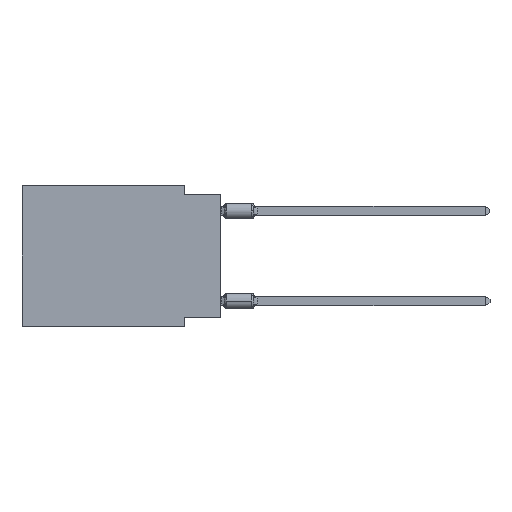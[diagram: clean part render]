
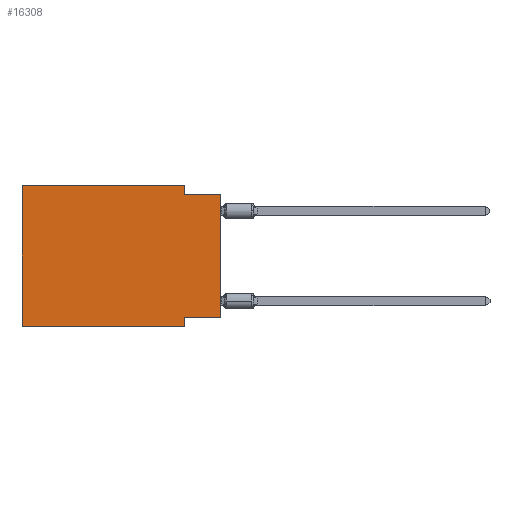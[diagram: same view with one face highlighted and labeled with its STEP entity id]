
A CAD part, left-side view. The second image highlights one B-rep face of the part: STEP entity #16308.
In plain terms, the highlighted planar face has unit normal (-1, 0, 0).
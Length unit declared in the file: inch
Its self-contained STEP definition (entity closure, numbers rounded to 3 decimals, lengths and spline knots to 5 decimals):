
#1182 = VERTEX_POINT ( 'NONE', #14767 ) ;
#1268 = AXIS2_PLACEMENT_3D ( 'NONE', #7050, #26869, #10856 ) ;
#2631 = DIRECTION ( 'NONE',  ( 0., 0., -1. ) ) ;
#3006 = EDGE_CURVE ( 'NONE', #36230, #23345, #48469, .T. ) ;
#3013 = LINE ( 'NONE', #48326, #14189 ) ;
#3287 = CARTESIAN_POINT ( 'NONE',  ( 0., 0.1, -0.39 ) ) ;
#4410 = CARTESIAN_POINT ( 'NONE',  ( 0., 0.1, -0.025 ) ) ;
#4413 = ORIENTED_EDGE ( 'NONE', *, *, #25421, .F. ) ;
#4939 = DIRECTION ( 'NONE',  ( 0., -1., 0. ) ) ;
#4994 = VERTEX_POINT ( 'NONE', #48086 ) ;
#7050 = CARTESIAN_POINT ( 'NONE',  ( 0., 0.55, 0. ) ) ;
#7879 = ORIENTED_EDGE ( 'NONE', *, *, #24245, .F. ) ;
#8689 = CARTESIAN_POINT ( 'NONE',  ( 0., 0.55, -0.39 ) ) ;
#9275 = CARTESIAN_POINT ( 'NONE',  ( 0., 0., -0.365 ) ) ;
#10856 = DIRECTION ( 'NONE',  ( 0., 0., -1. ) ) ;
#10916 = VECTOR ( 'NONE', #2631, 39.37008 ) ;
#11179 = CARTESIAN_POINT ( 'NONE',  ( 0., 0.1, -0.39 ) ) ;
#14189 = VECTOR ( 'NONE', #52661, 39.37008 ) ;
#14614 = VERTEX_POINT ( 'NONE', #11179 ) ;
#14627 = EDGE_LOOP ( 'NONE', ( #42340, #7879, #46774, #4413, #25783, #42795, #32193, #40456 ) ) ;
#14767 = CARTESIAN_POINT ( 'NONE',  ( 0., 0., -0.365 ) ) ;
#16308 = ADVANCED_FACE ( 'NONE', ( #47497 ), #23058, .F. ) ;
#16855 = DIRECTION ( 'NONE',  ( 0., 1., 0. ) ) ;
#17126 = LINE ( 'NONE', #9275, #35030 ) ;
#19796 = EDGE_CURVE ( 'NONE', #1182, #48829, #17126, .T. ) ;
#21618 = LINE ( 'NONE', #33315, #40426 ) ;
#23058 = PLANE ( 'NONE',  #1268 ) ;
#23190 = DIRECTION ( 'NONE',  ( 0., 0., 1. ) ) ;
#23345 = VERTEX_POINT ( 'NONE', #4410 ) ;
#24245 = EDGE_CURVE ( 'NONE', #23345, #4994, #21618, .T. ) ;
#24472 = VECTOR ( 'NONE', #49923, 39.37008 ) ;
#24552 = VERTEX_POINT ( 'NONE', #31359 ) ;
#25267 = LINE ( 'NONE', #42107, #45704 ) ;
#25421 = EDGE_CURVE ( 'NONE', #49332, #36230, #25267, .T. ) ;
#25695 = DIRECTION ( 'NONE',  ( 0., -1., 0. ) ) ;
#25783 = ORIENTED_EDGE ( 'NONE', *, *, #34058, .F. ) ;
#26869 = DIRECTION ( 'NONE',  ( 1., 0., 0. ) ) ;
#27045 = CARTESIAN_POINT ( 'NONE',  ( 0., 0.1, 0. ) ) ;
#28345 = LINE ( 'NONE', #44614, #34108 ) ;
#28780 = DIRECTION ( 'NONE',  ( 0., 0., -1. ) ) ;
#29845 = LINE ( 'NONE', #8689, #24472 ) ;
#31359 = CARTESIAN_POINT ( 'NONE',  ( 0., 0.55, -0.39 ) ) ;
#32193 = ORIENTED_EDGE ( 'NONE', *, *, #51694, .F. ) ;
#33315 = CARTESIAN_POINT ( 'NONE',  ( 0., 0., -0.025 ) ) ;
#34058 = EDGE_CURVE ( 'NONE', #24552, #49332, #28345, .T. ) ;
#34108 = VECTOR ( 'NONE', #23190, 39.37008 ) ;
#35030 = VECTOR ( 'NONE', #16855, 39.37008 ) ;
#36230 = VERTEX_POINT ( 'NONE', #52368 ) ;
#36698 = CARTESIAN_POINT ( 'NONE',  ( 0., 0.1, -0.365 ) ) ;
#40426 = VECTOR ( 'NONE', #25695, 39.37008 ) ;
#40453 = LINE ( 'NONE', #3287, #51501 ) ;
#40456 = ORIENTED_EDGE ( 'NONE', *, *, #19796, .F. ) ;
#42107 = CARTESIAN_POINT ( 'NONE',  ( 0., 0.55, 0. ) ) ;
#42340 = ORIENTED_EDGE ( 'NONE', *, *, #51646, .T. ) ;
#42795 = ORIENTED_EDGE ( 'NONE', *, *, #50523, .T. ) ;
#44614 = CARTESIAN_POINT ( 'NONE',  ( 0., 0.55, 0. ) ) ;
#45704 = VECTOR ( 'NONE', #4939, 39.37008 ) ;
#46774 = ORIENTED_EDGE ( 'NONE', *, *, #3006, .F. ) ;
#47497 = FACE_OUTER_BOUND ( 'NONE', #14627, .T. ) ;
#48086 = CARTESIAN_POINT ( 'NONE',  ( 0., 0., -0.025 ) ) ;
#48326 = CARTESIAN_POINT ( 'NONE',  ( 0., 0., 0. ) ) ;
#48469 = LINE ( 'NONE', #27045, #10916 ) ;
#48829 = VERTEX_POINT ( 'NONE', #36698 ) ;
#49332 = VERTEX_POINT ( 'NONE', #53438 ) ;
#49923 = DIRECTION ( 'NONE',  ( 0., -1., 0. ) ) ;
#50523 = EDGE_CURVE ( 'NONE', #24552, #14614, #29845, .T. ) ;
#51501 = VECTOR ( 'NONE', #28780, 39.37008 ) ;
#51646 = EDGE_CURVE ( 'NONE', #1182, #4994, #3013, .T. ) ;
#51694 = EDGE_CURVE ( 'NONE', #48829, #14614, #40453, .T. ) ;
#52368 = CARTESIAN_POINT ( 'NONE',  ( 0., 0.1, 0. ) ) ;
#52661 = DIRECTION ( 'NONE',  ( 0., 0., 1. ) ) ;
#53438 = CARTESIAN_POINT ( 'NONE',  ( 0., 0.55, 0. ) ) ;
